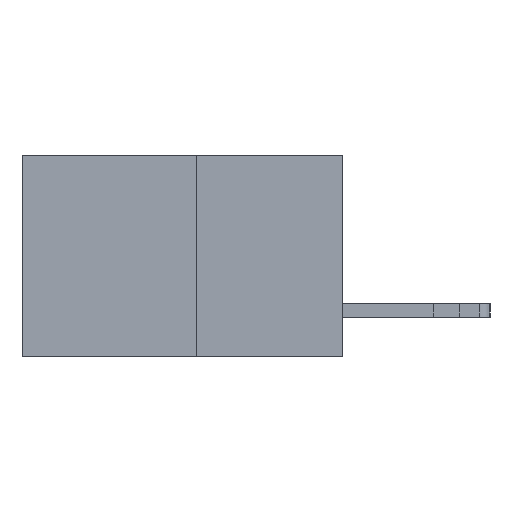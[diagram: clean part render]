
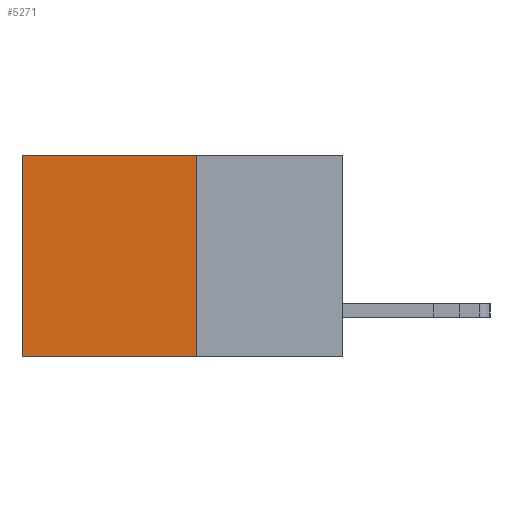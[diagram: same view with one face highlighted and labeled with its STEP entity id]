
A CAD part, left-side view. The second image highlights one B-rep face of the part: STEP entity #5271.
In plain terms, the highlighted planar face has unit normal (-1, 0, 0).
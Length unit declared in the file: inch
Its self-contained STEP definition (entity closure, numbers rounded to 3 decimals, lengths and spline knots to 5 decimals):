
#528 = PLANE ( 'NONE',  #6358 ) ;
#550 = EDGE_CURVE ( 'NONE', #10503, #5721, #5770, .T. ) ;
#1491 = VERTEX_POINT ( 'NONE', #2875 ) ;
#1620 = CARTESIAN_POINT ( 'NONE',  ( 0.277, 0.27, -0.37 ) ) ;
#2045 = DIRECTION ( 'NONE',  ( 0., 1., 0. ) ) ;
#2262 = EDGE_CURVE ( 'NONE', #1491, #10503, #10504, .T. ) ;
#2347 = VECTOR ( 'NONE', #5540, 39.37008 ) ;
#2359 = CARTESIAN_POINT ( 'NONE',  ( 0.277, 0.59, -0.37 ) ) ;
#2669 = DIRECTION ( 'NONE',  ( 0., 0., -1. ) ) ;
#2875 = CARTESIAN_POINT ( 'NONE',  ( 0.277, 0.27, 0. ) ) ;
#3128 = ORIENTED_EDGE ( 'NONE', *, *, #10215, .T. ) ;
#3211 = CARTESIAN_POINT ( 'NONE',  ( 0.277, 0.59, -0.37 ) ) ;
#3405 = DIRECTION ( 'NONE',  ( 0., 0., -1. ) ) ;
#5271 = ADVANCED_FACE ( 'NONE', ( #8090 ), #528, .F. ) ;
#5540 = DIRECTION ( 'NONE',  ( 0., 1., 0. ) ) ;
#5721 = VERTEX_POINT ( 'NONE', #3211 ) ;
#5770 = LINE ( 'NONE', #6578, #6431 ) ;
#5894 = CARTESIAN_POINT ( 'NONE',  ( 0.277, 0.27, -0.37 ) ) ;
#6139 = VECTOR ( 'NONE', #3405, 39.37008 ) ;
#6358 = AXIS2_PLACEMENT_3D ( 'NONE', #1620, #9012, #2669 ) ;
#6431 = VECTOR ( 'NONE', #2045, 39.37008 ) ;
#6578 = CARTESIAN_POINT ( 'NONE',  ( 0.277, 0.27, -0.37 ) ) ;
#6654 = ORIENTED_EDGE ( 'NONE', *, *, #10253, .T. ) ;
#7437 = EDGE_LOOP ( 'NONE', ( #3128, #10336, #12436, #6654 ) ) ;
#7611 = DIRECTION ( 'NONE',  ( 0., 0., -1. ) ) ;
#7843 = CARTESIAN_POINT ( 'NONE',  ( 0.277, 0.27, -0.37 ) ) ;
#8090 = FACE_OUTER_BOUND ( 'NONE', #7437, .T. ) ;
#8185 = CARTESIAN_POINT ( 'NONE',  ( 0.277, 0.59, 0. ) ) ;
#8299 = LINE ( 'NONE', #2359, #6139 ) ;
#8740 = CARTESIAN_POINT ( 'NONE',  ( 0.277, 0.27, 0. ) ) ;
#9012 = DIRECTION ( 'NONE',  ( 1., 0., 0. ) ) ;
#9861 = VECTOR ( 'NONE', #7611, 39.37008 ) ;
#9902 = VERTEX_POINT ( 'NONE', #8185 ) ;
#10215 = EDGE_CURVE ( 'NONE', #9902, #5721, #8299, .T. ) ;
#10253 = EDGE_CURVE ( 'NONE', #1491, #9902, #10765, .T. ) ;
#10336 = ORIENTED_EDGE ( 'NONE', *, *, #550, .F. ) ;
#10503 = VERTEX_POINT ( 'NONE', #5894 ) ;
#10504 = LINE ( 'NONE', #7843, #9861 ) ;
#10765 = LINE ( 'NONE', #8740, #2347 ) ;
#12436 = ORIENTED_EDGE ( 'NONE', *, *, #2262, .F. ) ;
